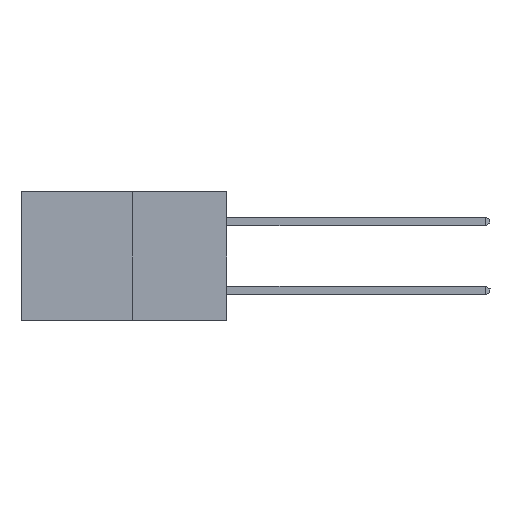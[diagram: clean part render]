
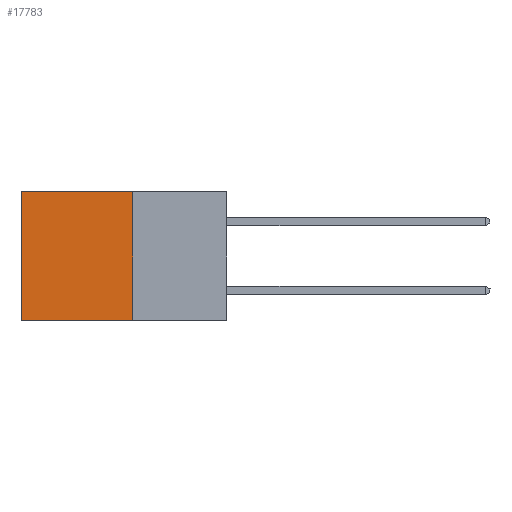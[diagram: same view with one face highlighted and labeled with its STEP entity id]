
A CAD part, left-side view. The second image highlights one B-rep face of the part: STEP entity #17783.
In plain terms, the highlighted planar face has unit normal (-1, 0, 0).
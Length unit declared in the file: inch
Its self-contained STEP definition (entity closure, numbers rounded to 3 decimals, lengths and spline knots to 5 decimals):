
#1531 = CARTESIAN_POINT ( 'NONE',  ( 0.277, 0.27, -0.37 ) ) ;
#2331 = VECTOR ( 'NONE', #35741, 39.37008 ) ;
#3330 = DIRECTION ( 'NONE',  ( 0., 0., -1. ) ) ;
#3787 = LINE ( 'NONE', #6458, #25820 ) ;
#4407 = DIRECTION ( 'NONE',  ( 1., 0., 0. ) ) ;
#6458 = CARTESIAN_POINT ( 'NONE',  ( 0.277, 0.27, 0. ) ) ;
#6816 = EDGE_CURVE ( 'NONE', #8293, #27183, #3787, .T. ) ;
#8061 = ORIENTED_EDGE ( 'NONE', *, *, #19567, .T. ) ;
#8293 = VERTEX_POINT ( 'NONE', #18162 ) ;
#8378 = FACE_OUTER_BOUND ( 'NONE', #9162, .T. ) ;
#8703 = EDGE_CURVE ( 'NONE', #8293, #26015, #9889, .T. ) ;
#9162 = EDGE_LOOP ( 'NONE', ( #8061, #34647, #19533, #9373 ) ) ;
#9373 = ORIENTED_EDGE ( 'NONE', *, *, #6816, .T. ) ;
#9889 = LINE ( 'NONE', #11462, #23061 ) ;
#9967 = CARTESIAN_POINT ( 'NONE',  ( 0.277, 0.27, -0.37 ) ) ;
#10345 = CARTESIAN_POINT ( 'NONE',  ( 0.277, 0.59, 0. ) ) ;
#11408 = LINE ( 'NONE', #28478, #32751 ) ;
#11462 = CARTESIAN_POINT ( 'NONE',  ( 0.277, 0.27, -0.37 ) ) ;
#12075 = AXIS2_PLACEMENT_3D ( 'NONE', #9967, #4407, #24098 ) ;
#13930 = EDGE_CURVE ( 'NONE', #26015, #16956, #32944, .T. ) ;
#16956 = VERTEX_POINT ( 'NONE', #30843 ) ;
#17783 = ADVANCED_FACE ( 'NONE', ( #8378 ), #35040, .F. ) ;
#18162 = CARTESIAN_POINT ( 'NONE',  ( 0.277, 0.27, 0. ) ) ;
#19533 = ORIENTED_EDGE ( 'NONE', *, *, #8703, .F. ) ;
#19567 = EDGE_CURVE ( 'NONE', #27183, #16956, #11408, .T. ) ;
#21855 = CARTESIAN_POINT ( 'NONE',  ( 0.277, 0.27, -0.37 ) ) ;
#23061 = VECTOR ( 'NONE', #33725, 39.37008 ) ;
#24098 = DIRECTION ( 'NONE',  ( 0., 0., -1. ) ) ;
#25820 = VECTOR ( 'NONE', #31646, 39.37008 ) ;
#26015 = VERTEX_POINT ( 'NONE', #1531 ) ;
#27183 = VERTEX_POINT ( 'NONE', #10345 ) ;
#28478 = CARTESIAN_POINT ( 'NONE',  ( 0.277, 0.59, -0.37 ) ) ;
#30843 = CARTESIAN_POINT ( 'NONE',  ( 0.277, 0.59, -0.37 ) ) ;
#31646 = DIRECTION ( 'NONE',  ( 0., 1., 0. ) ) ;
#32751 = VECTOR ( 'NONE', #3330, 39.37008 ) ;
#32944 = LINE ( 'NONE', #21855, #2331 ) ;
#33725 = DIRECTION ( 'NONE',  ( 0., 0., -1. ) ) ;
#34647 = ORIENTED_EDGE ( 'NONE', *, *, #13930, .F. ) ;
#35040 = PLANE ( 'NONE',  #12075 ) ;
#35741 = DIRECTION ( 'NONE',  ( 0., 1., 0. ) ) ;
